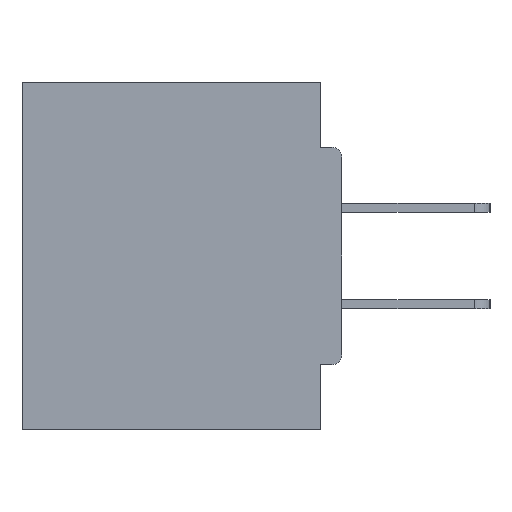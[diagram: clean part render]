
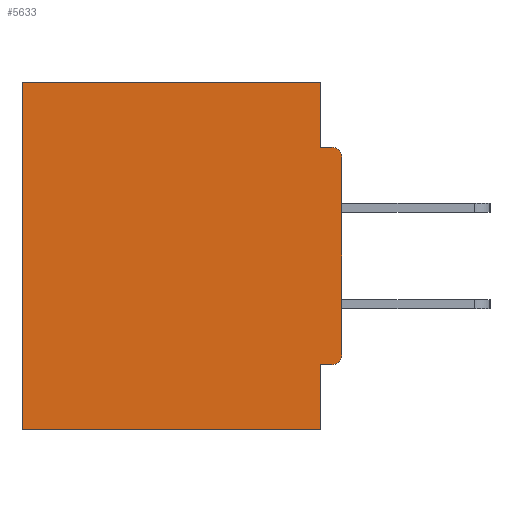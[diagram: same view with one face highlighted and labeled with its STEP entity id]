
A CAD part, left-side view. The second image highlights one B-rep face of the part: STEP entity #5633.
In plain terms, the highlighted planar face has unit normal (-1, 0, 0).
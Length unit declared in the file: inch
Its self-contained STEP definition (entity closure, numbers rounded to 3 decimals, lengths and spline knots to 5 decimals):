
#40 = CARTESIAN_POINT ( 'NONE',  ( 0.298, 0.031, -0.5 ) ) ;
#332 = CARTESIAN_POINT ( 'NONE',  ( 0.298, 0., 0. ) ) ;
#531 = CIRCLE ( 'NONE', #26396, 0.015 ) ;
#802 = CARTESIAN_POINT ( 'NONE',  ( 0.298, 0.031, -0.5 ) ) ;
#873 = DIRECTION ( 'NONE',  ( 0., 0., -1. ) ) ;
#1390 = DIRECTION ( 'NONE',  ( 0., 0., -1. ) ) ;
#1583 = ORIENTED_EDGE ( 'NONE', *, *, #26680, .F. ) ;
#1866 = ORIENTED_EDGE ( 'NONE', *, *, #10679, .F. ) ;
#1878 = DIRECTION ( 'NONE',  ( -1., 0., 0. ) ) ;
#2123 = EDGE_CURVE ( 'NONE', #10491, #14093, #11302, .T. ) ;
#2181 = DIRECTION ( 'NONE',  ( 0., 1., 0. ) ) ;
#4817 = VECTOR ( 'NONE', #22308, 39.37008 ) ;
#4880 = ORIENTED_EDGE ( 'NONE', *, *, #5487, .F. ) ;
#5487 = EDGE_CURVE ( 'NONE', #18800, #32269, #23591, .T. ) ;
#5633 = ADVANCED_FACE ( 'NONE', ( #25193 ), #29271, .F. ) ;
#6248 = LINE ( 'NONE', #802, #11475 ) ;
#6268 = CARTESIAN_POINT ( 'NONE',  ( 0.298, 0.015, -0.1085 ) ) ;
#6295 = CARTESIAN_POINT ( 'NONE',  ( 0.298, 0., -0.1085 ) ) ;
#7047 = CARTESIAN_POINT ( 'NONE',  ( 0.298, 0., -0.4065 ) ) ;
#8117 = DIRECTION ( 'NONE',  ( 0., 0., -1. ) ) ;
#8411 = EDGE_CURVE ( 'NONE', #12450, #10292, #22714, .T. ) ;
#8583 = VECTOR ( 'NONE', #28603, 39.37008 ) ;
#9799 = ORIENTED_EDGE ( 'NONE', *, *, #2123, .F. ) ;
#9911 = DIRECTION ( 'NONE',  ( 0., 0., -1. ) ) ;
#10112 = CARTESIAN_POINT ( 'NONE',  ( 0.298, 0.031, 0. ) ) ;
#10292 = VERTEX_POINT ( 'NONE', #22576 ) ;
#10432 = LINE ( 'NONE', #26847, #26641 ) ;
#10491 = VERTEX_POINT ( 'NONE', #15755 ) ;
#10679 = EDGE_CURVE ( 'NONE', #14093, #10878, #20898, .T. ) ;
#10878 = VERTEX_POINT ( 'NONE', #17445 ) ;
#11302 = LINE ( 'NONE', #30030, #4817 ) ;
#11475 = VECTOR ( 'NONE', #24432, 39.37008 ) ;
#11918 = ORIENTED_EDGE ( 'NONE', *, *, #30839, .F. ) ;
#12450 = VERTEX_POINT ( 'NONE', #10112 ) ;
#12641 = CARTESIAN_POINT ( 'NONE',  ( 0.298, 0., 0. ) ) ;
#12720 = VERTEX_POINT ( 'NONE', #28406 ) ;
#13584 = ORIENTED_EDGE ( 'NONE', *, *, #19628, .T. ) ;
#14007 = VECTOR ( 'NONE', #18948, 39.37008 ) ;
#14093 = VERTEX_POINT ( 'NONE', #40 ) ;
#14253 = AXIS2_PLACEMENT_3D ( 'NONE', #31778, #16137, #873 ) ;
#14765 = CARTESIAN_POINT ( 'NONE',  ( 0.298, 0.015, -0.0935 ) ) ;
#15241 = DIRECTION ( 'NONE',  ( 0., 1., 0. ) ) ;
#15755 = CARTESIAN_POINT ( 'NONE',  ( 0.298, 0.031, -0.4065 ) ) ;
#16137 = DIRECTION ( 'NONE',  ( 1., 0., 0. ) ) ;
#16619 = VECTOR ( 'NONE', #15241, 39.37008 ) ;
#17062 = LINE ( 'NONE', #17520, #8583 ) ;
#17445 = CARTESIAN_POINT ( 'NONE',  ( 0.298, 0.46, -0.5 ) ) ;
#17520 = CARTESIAN_POINT ( 'NONE',  ( 0.298, 0.46, 0. ) ) ;
#17570 = AXIS2_PLACEMENT_3D ( 'NONE', #30416, #1878, #9911 ) ;
#17829 = VECTOR ( 'NONE', #2181, 39.37008 ) ;
#18343 = VECTOR ( 'NONE', #8117, 39.37008 ) ;
#18800 = VERTEX_POINT ( 'NONE', #6295 ) ;
#18948 = DIRECTION ( 'NONE',  ( 0., 1., 0. ) ) ;
#19055 = CARTESIAN_POINT ( 'NONE',  ( 0.298, 0., -0.5 ) ) ;
#19162 = DIRECTION ( 'NONE',  ( 0., -1., 0. ) ) ;
#19628 = EDGE_CURVE ( 'NONE', #12720, #32269, #31875, .T. ) ;
#19767 = CARTESIAN_POINT ( 'NONE',  ( 0.298, 0., -0.3915 ) ) ;
#20898 = LINE ( 'NONE', #19055, #14007 ) ;
#22308 = DIRECTION ( 'NONE',  ( 0., 0., -1. ) ) ;
#22518 = EDGE_CURVE ( 'NONE', #10292, #10878, #17062, .T. ) ;
#22576 = CARTESIAN_POINT ( 'NONE',  ( 0.298, 0.46, 0. ) ) ;
#22714 = LINE ( 'NONE', #12641, #16619 ) ;
#23095 = ORIENTED_EDGE ( 'NONE', *, *, #27419, .T. ) ;
#23544 = VERTEX_POINT ( 'NONE', #14765 ) ;
#23591 = LINE ( 'NONE', #332, #18343 ) ;
#23926 = EDGE_CURVE ( 'NONE', #12720, #10491, #25093, .T. ) ;
#24117 = VERTEX_POINT ( 'NONE', #31054 ) ;
#24369 = DIRECTION ( 'NONE',  ( -1., 0., 0. ) ) ;
#24432 = DIRECTION ( 'NONE',  ( 0., 0., -1. ) ) ;
#25093 = LINE ( 'NONE', #7047, #17829 ) ;
#25193 = FACE_OUTER_BOUND ( 'NONE', #30228, .T. ) ;
#26396 = AXIS2_PLACEMENT_3D ( 'NONE', #6268, #24369, #1390 ) ;
#26641 = VECTOR ( 'NONE', #19162, 39.37008 ) ;
#26680 = EDGE_CURVE ( 'NONE', #12450, #24117, #6248, .T. ) ;
#26847 = CARTESIAN_POINT ( 'NONE',  ( 0.298, 0., -0.0935 ) ) ;
#26987 = ORIENTED_EDGE ( 'NONE', *, *, #22518, .T. ) ;
#27419 = EDGE_CURVE ( 'NONE', #18800, #23544, #531, .T. ) ;
#28406 = CARTESIAN_POINT ( 'NONE',  ( 0.298, 0.015, -0.4065 ) ) ;
#28452 = ORIENTED_EDGE ( 'NONE', *, *, #23926, .F. ) ;
#28603 = DIRECTION ( 'NONE',  ( 0., 0., -1. ) ) ;
#29271 = PLANE ( 'NONE',  #14253 ) ;
#30030 = CARTESIAN_POINT ( 'NONE',  ( 0.298, 0.031, -0.5 ) ) ;
#30228 = EDGE_LOOP ( 'NONE', ( #23095, #11918, #1583, #32394, #26987, #1866, #9799, #28452, #13584, #4880 ) ) ;
#30416 = CARTESIAN_POINT ( 'NONE',  ( 0.298, 0.015, -0.3915 ) ) ;
#30839 = EDGE_CURVE ( 'NONE', #24117, #23544, #10432, .T. ) ;
#31054 = CARTESIAN_POINT ( 'NONE',  ( 0.298, 0.031, -0.0935 ) ) ;
#31778 = CARTESIAN_POINT ( 'NONE',  ( 0.298, 0., 0. ) ) ;
#31875 = CIRCLE ( 'NONE', #17570, 0.015 ) ;
#32269 = VERTEX_POINT ( 'NONE', #19767 ) ;
#32394 = ORIENTED_EDGE ( 'NONE', *, *, #8411, .T. ) ;
